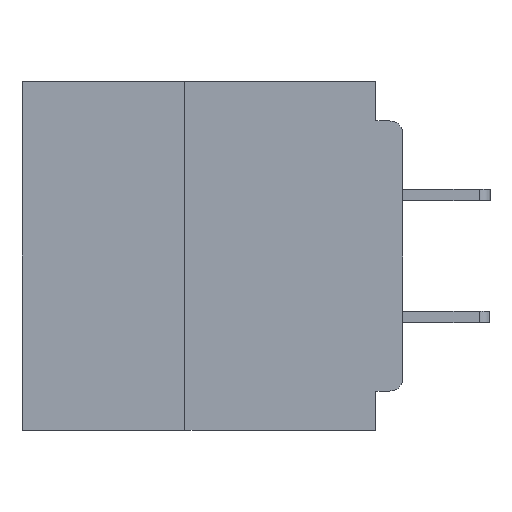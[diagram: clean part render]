
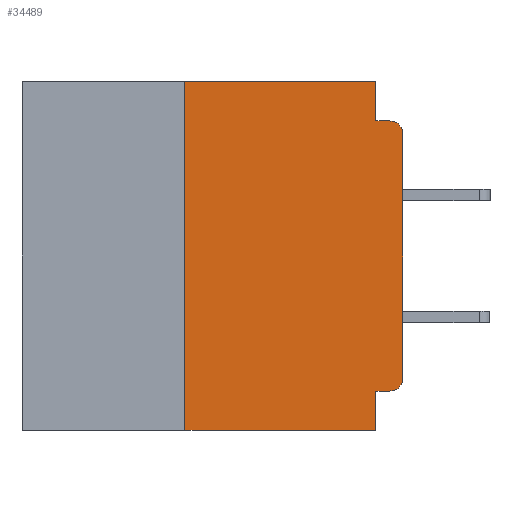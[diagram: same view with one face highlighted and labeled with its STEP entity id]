
A CAD part, left-side view. The second image highlights one B-rep face of the part: STEP entity #34489.
In plain terms, the highlighted planar face has unit normal (-1, 0, 0).
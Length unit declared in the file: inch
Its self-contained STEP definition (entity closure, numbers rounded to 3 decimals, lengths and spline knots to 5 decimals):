
#1121 = CARTESIAN_POINT ( 'NONE',  ( 0., 0.25, 0. ) ) ;
#1482 = ORIENTED_EDGE ( 'NONE', *, *, #28840, .T. ) ;
#1798 = DIRECTION ( 'NONE',  ( 0., -1., 0. ) ) ;
#2006 = VERTEX_POINT ( 'NONE', #10760 ) ;
#2116 = CARTESIAN_POINT ( 'NONE',  ( 0., 0.015, -0.06 ) ) ;
#2468 = DIRECTION ( 'NONE',  ( -1., 0., 0. ) ) ;
#3135 = LINE ( 'NONE', #39200, #11409 ) ;
#3933 = CARTESIAN_POINT ( 'NONE',  ( 0., 0., -0.34 ) ) ;
#4264 = ORIENTED_EDGE ( 'NONE', *, *, #19425, .F. ) ;
#4680 = EDGE_CURVE ( 'NONE', #33839, #32574, #18564, .T. ) ;
#4765 = CARTESIAN_POINT ( 'NONE',  ( 0., 0., 0. ) ) ;
#4928 = DIRECTION ( 'NONE',  ( 0., 0., 1. ) ) ;
#4966 = VECTOR ( 'NONE', #18380, 39.37008 ) ;
#5290 = AXIS2_PLACEMENT_3D ( 'NONE', #23296, #2468, #26702 ) ;
#5710 = DIRECTION ( 'NONE',  ( 0., 0., -1. ) ) ;
#7603 = ORIENTED_EDGE ( 'NONE', *, *, #36392, .F. ) ;
#8280 = VECTOR ( 'NONE', #4928, 39.37008 ) ;
#8607 = LINE ( 'NONE', #25986, #43007 ) ;
#8633 = CARTESIAN_POINT ( 'NONE',  ( 0., 0.031, 0. ) ) ;
#10452 = LINE ( 'NONE', #43190, #27616 ) ;
#10760 = CARTESIAN_POINT ( 'NONE',  ( 0., 0.25, -0.4 ) ) ;
#11132 = AXIS2_PLACEMENT_3D ( 'NONE', #2116, #26381, #5710 ) ;
#11409 = VECTOR ( 'NONE', #42626, 39.37008 ) ;
#12502 = ORIENTED_EDGE ( 'NONE', *, *, #18624, .F. ) ;
#12928 = DIRECTION ( 'NONE',  ( 0., 0., -1. ) ) ;
#13932 = EDGE_CURVE ( 'NONE', #42286, #14755, #35661, .T. ) ;
#14755 = VERTEX_POINT ( 'NONE', #41959 ) ;
#14819 = CARTESIAN_POINT ( 'NONE',  ( 0., 0.015, -0.045 ) ) ;
#15669 = DIRECTION ( 'NONE',  ( 0., 0., -1. ) ) ;
#16954 = CARTESIAN_POINT ( 'NONE',  ( 0., 0., -0.06 ) ) ;
#17897 = DIRECTION ( 'NONE',  ( 1., 0., 0. ) ) ;
#18302 = EDGE_LOOP ( 'NONE', ( #44690, #18432, #12502, #21680, #4264, #7603, #1482, #38301, #21153, #33495 ) ) ;
#18380 = DIRECTION ( 'NONE',  ( 0., -1., 0. ) ) ;
#18432 = ORIENTED_EDGE ( 'NONE', *, *, #19362, .T. ) ;
#18564 = LINE ( 'NONE', #4765, #8280 ) ;
#18624 = EDGE_CURVE ( 'NONE', #14755, #38466, #32509, .T. ) ;
#19362 = EDGE_CURVE ( 'NONE', #32574, #38466, #30569, .T. ) ;
#19425 = EDGE_CURVE ( 'NONE', #29376, #42286, #34355, .T. ) ;
#20680 = VERTEX_POINT ( 'NONE', #33822 ) ;
#21153 = ORIENTED_EDGE ( 'NONE', *, *, #22597, .F. ) ;
#21680 = ORIENTED_EDGE ( 'NONE', *, *, #13932, .F. ) ;
#22597 = EDGE_CURVE ( 'NONE', #20680, #30119, #39475, .T. ) ;
#23158 = CARTESIAN_POINT ( 'NONE',  ( 0., 0.031, -0.355 ) ) ;
#23225 = EDGE_CURVE ( 'NONE', #20680, #33839, #25388, .T. ) ;
#23262 = DIRECTION ( 'NONE',  ( 0., -1., 0. ) ) ;
#23296 = CARTESIAN_POINT ( 'NONE',  ( 0., 0.015, -0.34 ) ) ;
#25388 = CIRCLE ( 'NONE', #5290, 0.015 ) ;
#25986 = CARTESIAN_POINT ( 'NONE',  ( 0., 0.031, -0.4 ) ) ;
#26381 = DIRECTION ( 'NONE',  ( -1., 0., 0. ) ) ;
#26702 = DIRECTION ( 'NONE',  ( 0., 0., -1. ) ) ;
#26759 = CARTESIAN_POINT ( 'NONE',  ( 0., 0., -0.355 ) ) ;
#27616 = VECTOR ( 'NONE', #1798, 39.37008 ) ;
#28043 = CARTESIAN_POINT ( 'NONE',  ( 0., 0.437, 0. ) ) ;
#28531 = CARTESIAN_POINT ( 'NONE',  ( 0., 0., -0.045 ) ) ;
#28628 = VECTOR ( 'NONE', #12928, 39.37008 ) ;
#28840 = EDGE_CURVE ( 'NONE', #2006, #36535, #10452, .T. ) ;
#29376 = VERTEX_POINT ( 'NONE', #1121 ) ;
#30119 = VERTEX_POINT ( 'NONE', #23158 ) ;
#30321 = VECTOR ( 'NONE', #40603, 39.37008 ) ;
#30569 = CIRCLE ( 'NONE', #11132, 0.015 ) ;
#32509 = LINE ( 'NONE', #28531, #4966 ) ;
#32574 = VERTEX_POINT ( 'NONE', #16954 ) ;
#33495 = ORIENTED_EDGE ( 'NONE', *, *, #23225, .T. ) ;
#33506 = CARTESIAN_POINT ( 'NONE',  ( 0., 0.031, 0. ) ) ;
#33822 = CARTESIAN_POINT ( 'NONE',  ( 0., 0.015, -0.355 ) ) ;
#33839 = VERTEX_POINT ( 'NONE', #3933 ) ;
#34355 = LINE ( 'NONE', #40369, #42386 ) ;
#34489 = ADVANCED_FACE ( 'NONE', ( #37399 ), #38441, .F. ) ;
#35661 = LINE ( 'NONE', #33506, #28628 ) ;
#36392 = EDGE_CURVE ( 'NONE', #2006, #29376, #3135, .T. ) ;
#36535 = VERTEX_POINT ( 'NONE', #39943 ) ;
#37399 = FACE_OUTER_BOUND ( 'NONE', #18302, .T. ) ;
#37426 = EDGE_CURVE ( 'NONE', #30119, #36535, #8607, .T. ) ;
#38301 = ORIENTED_EDGE ( 'NONE', *, *, #37426, .F. ) ;
#38441 = PLANE ( 'NONE',  #44247 ) ;
#38466 = VERTEX_POINT ( 'NONE', #14819 ) ;
#39200 = CARTESIAN_POINT ( 'NONE',  ( 0., 0.25, -0.4 ) ) ;
#39475 = LINE ( 'NONE', #26759, #30321 ) ;
#39943 = CARTESIAN_POINT ( 'NONE',  ( 0., 0.031, -0.4 ) ) ;
#40369 = CARTESIAN_POINT ( 'NONE',  ( 0., 0.437, 0. ) ) ;
#40603 = DIRECTION ( 'NONE',  ( 0., 1., 0. ) ) ;
#41867 = DIRECTION ( 'NONE',  ( 0., 0., -1. ) ) ;
#41959 = CARTESIAN_POINT ( 'NONE',  ( 0., 0.031, -0.045 ) ) ;
#42286 = VERTEX_POINT ( 'NONE', #8633 ) ;
#42386 = VECTOR ( 'NONE', #23262, 39.37008 ) ;
#42626 = DIRECTION ( 'NONE',  ( 0., 0., 1. ) ) ;
#43007 = VECTOR ( 'NONE', #15669, 39.37008 ) ;
#43190 = CARTESIAN_POINT ( 'NONE',  ( 0., 0.437, -0.4 ) ) ;
#44247 = AXIS2_PLACEMENT_3D ( 'NONE', #28043, #17897, #41867 ) ;
#44690 = ORIENTED_EDGE ( 'NONE', *, *, #4680, .T. ) ;
